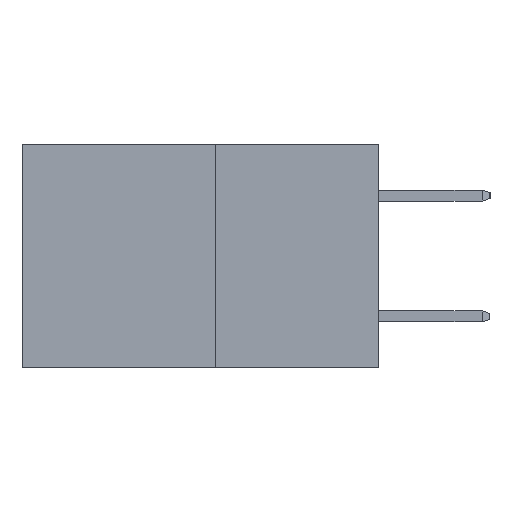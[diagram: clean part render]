
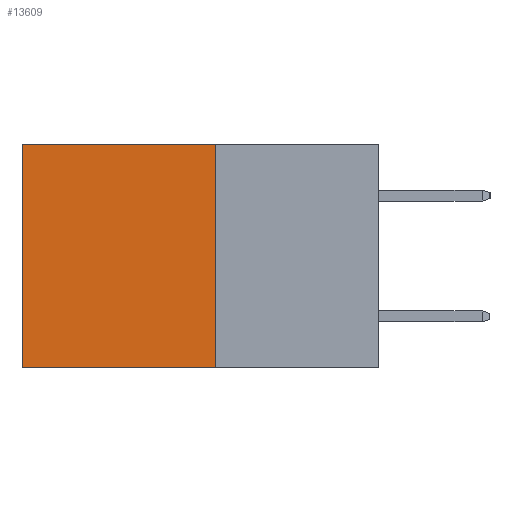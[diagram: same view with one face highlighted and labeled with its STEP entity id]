
A CAD part, left-side view. The second image highlights one B-rep face of the part: STEP entity #13609.
In plain terms, the highlighted planar face has unit normal (-1, 0, 0).
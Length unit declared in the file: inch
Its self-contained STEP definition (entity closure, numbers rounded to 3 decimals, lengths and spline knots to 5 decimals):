
#177 = LINE ( 'NONE', #15094, #4971 ) ;
#851 = EDGE_CURVE ( 'NONE', #15046, #11014, #21467, .T. ) ;
#3678 = FACE_OUTER_BOUND ( 'NONE', #8215, .T. ) ;
#4020 = VECTOR ( 'NONE', #13787, 39.37008 ) ;
#4054 = ORIENTED_EDGE ( 'NONE', *, *, #7622, .F. ) ;
#4543 = AXIS2_PLACEMENT_3D ( 'NONE', #14796, #16595, #5880 ) ;
#4971 = VECTOR ( 'NONE', #20315, 39.37008 ) ;
#5880 = DIRECTION ( 'NONE',  ( 0., 0., -1. ) ) ;
#6213 = CARTESIAN_POINT ( 'NONE',  ( 0.277, 0.27, 0. ) ) ;
#6777 = VECTOR ( 'NONE', #14580, 39.37008 ) ;
#7622 = EDGE_CURVE ( 'NONE', #11014, #8536, #17759, .T. ) ;
#8215 = EDGE_LOOP ( 'NONE', ( #16616, #4054, #8535, #22201 ) ) ;
#8356 = EDGE_CURVE ( 'NONE', #15046, #12220, #12171, .T. ) ;
#8535 = ORIENTED_EDGE ( 'NONE', *, *, #851, .F. ) ;
#8536 = VERTEX_POINT ( 'NONE', #14355 ) ;
#10391 = DIRECTION ( 'NONE',  ( 0., 1., 0. ) ) ;
#11014 = VERTEX_POINT ( 'NONE', #11247 ) ;
#11247 = CARTESIAN_POINT ( 'NONE',  ( 0.277, 0.27, -0.37 ) ) ;
#12171 = LINE ( 'NONE', #20966, #20468 ) ;
#12220 = VERTEX_POINT ( 'NONE', #19785 ) ;
#13016 = PLANE ( 'NONE',  #4543 ) ;
#13609 = ADVANCED_FACE ( 'NONE', ( #3678 ), #13016, .F. ) ;
#13787 = DIRECTION ( 'NONE',  ( 0., 1., 0. ) ) ;
#14355 = CARTESIAN_POINT ( 'NONE',  ( 0.277, 0.59, -0.37 ) ) ;
#14580 = DIRECTION ( 'NONE',  ( 0., 0., -1. ) ) ;
#14796 = CARTESIAN_POINT ( 'NONE',  ( 0.277, 0.27, -0.37 ) ) ;
#15046 = VERTEX_POINT ( 'NONE', #6213 ) ;
#15094 = CARTESIAN_POINT ( 'NONE',  ( 0.277, 0.59, -0.37 ) ) ;
#16415 = EDGE_CURVE ( 'NONE', #12220, #8536, #177, .T. ) ;
#16595 = DIRECTION ( 'NONE',  ( 1., 0., 0. ) ) ;
#16616 = ORIENTED_EDGE ( 'NONE', *, *, #16415, .T. ) ;
#17759 = LINE ( 'NONE', #22508, #4020 ) ;
#18060 = CARTESIAN_POINT ( 'NONE',  ( 0.277, 0.27, -0.37 ) ) ;
#19785 = CARTESIAN_POINT ( 'NONE',  ( 0.277, 0.59, 0. ) ) ;
#20315 = DIRECTION ( 'NONE',  ( 0., 0., -1. ) ) ;
#20468 = VECTOR ( 'NONE', #10391, 39.37008 ) ;
#20966 = CARTESIAN_POINT ( 'NONE',  ( 0.277, 0.27, 0. ) ) ;
#21467 = LINE ( 'NONE', #18060, #6777 ) ;
#22201 = ORIENTED_EDGE ( 'NONE', *, *, #8356, .T. ) ;
#22508 = CARTESIAN_POINT ( 'NONE',  ( 0.277, 0.27, -0.37 ) ) ;
